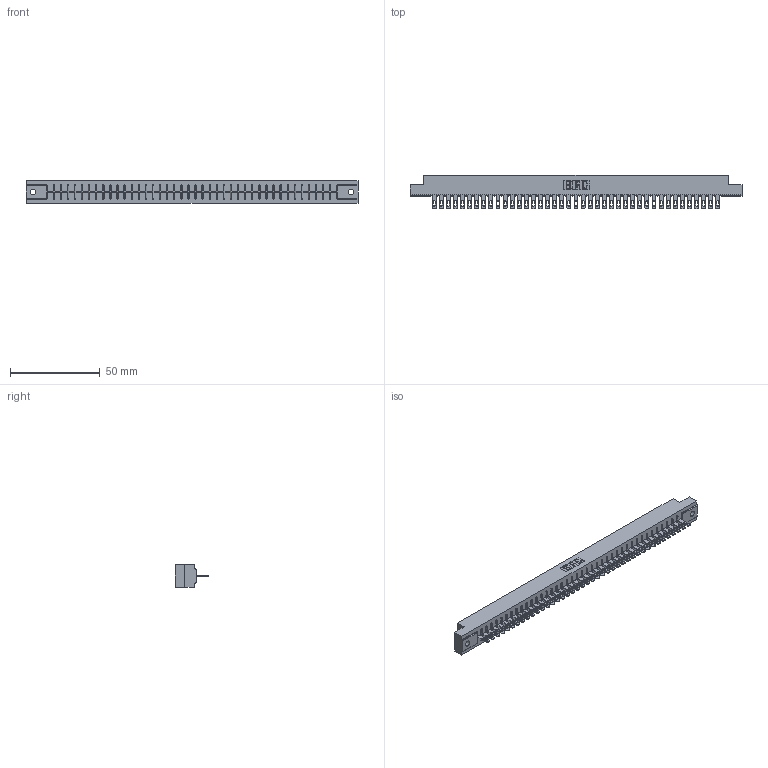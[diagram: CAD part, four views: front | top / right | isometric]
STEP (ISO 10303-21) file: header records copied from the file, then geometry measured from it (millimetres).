
FILE_DESCRIPTION (( 'STEP AP203' ), '1' );
FILE_NAME ('316-041-500-102.STEP', '2018-07-31T05:28:50', ( '' ), ( '' ), 'SwSTEP 2.0', 'SolidWorks 2016', '' );
FILE_SCHEMA (( 'CONFIG_CONTROL_DESIGN' ));
Length unit declared in the file: inch
Products named in the file (3): 306 Part_.128 Dia; 306-290-001_100; 316-041-500-102
Assembly tree (42 placements, depth 2):
  316-041-500-102
    306 Part_.128 Dia
    306-290-001_100  x41
Bounding box: 185.47 x 18.87 x 12.7 mm (x, y, z)
Volume: 20605.1 mm3; surface area: 21571.5 mm2
Topology: 42 solids, 42 shells, 3232 faces, 9131 edges, 5866 vertices
Faces by surface type: plane 2118, cylinder 950, sphere 164
Entity records: 38530 total; most frequent: CARTESIAN_POINT 6470, ORIENTED_EDGE 6414, DIRECTION 6381, EDGE_CURVE 3207, LINE 2507, VECTOR 2507, VERTEX_POINT 2026, AXIS2_PLACEMENT_3D 1937
